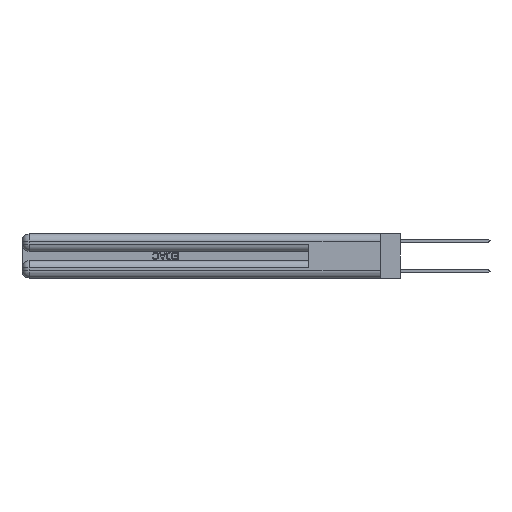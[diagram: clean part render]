
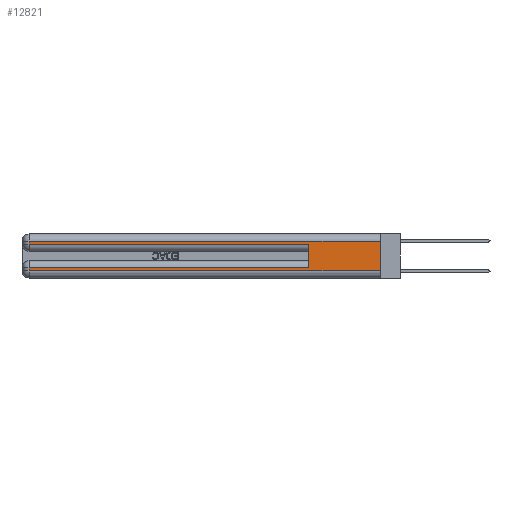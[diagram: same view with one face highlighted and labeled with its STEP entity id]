
A CAD part, left-side view. The second image highlights one B-rep face of the part: STEP entity #12821.
In plain terms, the highlighted planar face has unit normal (-1, 0, 0).
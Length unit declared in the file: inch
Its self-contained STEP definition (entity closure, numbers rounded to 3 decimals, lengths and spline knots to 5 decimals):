
#1538 = ORIENTED_EDGE ( 'NONE', *, *, #4470, .T. ) ;
#2518 = VERTEX_POINT ( 'NONE', #23135 ) ;
#2861 = VERTEX_POINT ( 'NONE', #29656 ) ;
#4069 = CARTESIAN_POINT ( 'NONE',  ( 0., 0., 0.06 ) ) ;
#4330 = DIRECTION ( 'NONE',  ( 0., -1., 0. ) ) ;
#4470 = EDGE_CURVE ( 'NONE', #31781, #13910, #30296, .T. ) ;
#4513 = CARTESIAN_POINT ( 'NONE',  ( 0., 0., 0.285 ) ) ;
#5048 = ORIENTED_EDGE ( 'NONE', *, *, #10285, .T. ) ;
#5128 = CARTESIAN_POINT ( 'NONE',  ( 0., 0., 0.06 ) ) ;
#5251 = ORIENTED_EDGE ( 'NONE', *, *, #26591, .F. ) ;
#5492 = DIRECTION ( 'NONE',  ( 0., 0., -1. ) ) ;
#5793 = ORIENTED_EDGE ( 'NONE', *, *, #26424, .T. ) ;
#5975 = FACE_OUTER_BOUND ( 'NONE', #10445, .T. ) ;
#6087 = LINE ( 'NONE', #33367, #21964 ) ;
#6448 = DIRECTION ( 'NONE',  ( 0., 1., 0. ) ) ;
#7720 = CARTESIAN_POINT ( 'NONE',  ( 0., 2.94, 0.31 ) ) ;
#8458 = PLANE ( 'NONE',  #12967 ) ;
#8974 = CARTESIAN_POINT ( 'NONE',  ( 0., 0.6, 0.285 ) ) ;
#8995 = EDGE_CURVE ( 'NONE', #2518, #31781, #30570, .T. ) ;
#9068 = EDGE_CURVE ( 'NONE', #13910, #26732, #9793, .T. ) ;
#9234 = CARTESIAN_POINT ( 'NONE',  ( 0., 0.6, 0.085 ) ) ;
#9793 = LINE ( 'NONE', #4513, #30836 ) ;
#10277 = EDGE_CURVE ( 'NONE', #2861, #21350, #22102, .T. ) ;
#10285 = EDGE_CURVE ( 'NONE', #30242, #2861, #6087, .T. ) ;
#10440 = DIRECTION ( 'NONE',  ( 0., 0., 1. ) ) ;
#10445 = EDGE_LOOP ( 'NONE', ( #5251, #25486, #1538, #22451, #24078, #5048, #30577, #5793 ) ) ;
#11769 = CARTESIAN_POINT ( 'NONE',  ( 0., 0., 0.37 ) ) ;
#12229 = CARTESIAN_POINT ( 'NONE',  ( 0., 2.94, 0.285 ) ) ;
#12821 = ADVANCED_FACE ( 'NONE', ( #5975 ), #8458, .F. ) ;
#12967 = AXIS2_PLACEMENT_3D ( 'NONE', #11769, #33254, #13726 ) ;
#13726 = DIRECTION ( 'NONE',  ( 0., 0., -1. ) ) ;
#13910 = VERTEX_POINT ( 'NONE', #12229 ) ;
#15384 = VECTOR ( 'NONE', #10440, 39.37008 ) ;
#15757 = EDGE_CURVE ( 'NONE', #30242, #26732, #32096, .T. ) ;
#16814 = DIRECTION ( 'NONE',  ( 0., 1., 0. ) ) ;
#17155 = DIRECTION ( 'NONE',  ( 0., 0., -1. ) ) ;
#17459 = VERTEX_POINT ( 'NONE', #5128 ) ;
#18529 = CARTESIAN_POINT ( 'NONE',  ( 0., 0.6, 0.145 ) ) ;
#20287 = VECTOR ( 'NONE', #23430, 39.37008 ) ;
#20439 = DIRECTION ( 'NONE',  ( 0., -1., 0. ) ) ;
#21315 = CARTESIAN_POINT ( 'NONE',  ( 0., 0., 0.37 ) ) ;
#21350 = VERTEX_POINT ( 'NONE', #24193 ) ;
#21964 = VECTOR ( 'NONE', #16814, 39.37008 ) ;
#22102 = LINE ( 'NONE', #30213, #33785 ) ;
#22451 = ORIENTED_EDGE ( 'NONE', *, *, #9068, .T. ) ;
#22723 = LINE ( 'NONE', #4069, #30981 ) ;
#22940 = VECTOR ( 'NONE', #6448, 39.37008 ) ;
#23135 = CARTESIAN_POINT ( 'NONE',  ( 0., 0., 0.31 ) ) ;
#23430 = DIRECTION ( 'NONE',  ( 0., 0., -1. ) ) ;
#23971 = LINE ( 'NONE', #21315, #20287 ) ;
#24078 = ORIENTED_EDGE ( 'NONE', *, *, #15757, .F. ) ;
#24193 = CARTESIAN_POINT ( 'NONE',  ( 0., 2.94, 0.06 ) ) ;
#25472 = CARTESIAN_POINT ( 'NONE',  ( 0., 0., 0.31 ) ) ;
#25486 = ORIENTED_EDGE ( 'NONE', *, *, #8995, .T. ) ;
#26424 = EDGE_CURVE ( 'NONE', #21350, #17459, #22723, .T. ) ;
#26591 = EDGE_CURVE ( 'NONE', #2518, #17459, #23971, .T. ) ;
#26732 = VERTEX_POINT ( 'NONE', #8974 ) ;
#29116 = VECTOR ( 'NONE', #5492, 39.37008 ) ;
#29622 = CARTESIAN_POINT ( 'NONE',  ( 0., 2.94, 0.37 ) ) ;
#29656 = CARTESIAN_POINT ( 'NONE',  ( 0., 2.94, 0.085 ) ) ;
#30213 = CARTESIAN_POINT ( 'NONE',  ( 0., 2.94, 0.37 ) ) ;
#30242 = VERTEX_POINT ( 'NONE', #9234 ) ;
#30296 = LINE ( 'NONE', #29622, #29116 ) ;
#30570 = LINE ( 'NONE', #25472, #22940 ) ;
#30577 = ORIENTED_EDGE ( 'NONE', *, *, #10277, .T. ) ;
#30836 = VECTOR ( 'NONE', #4330, 39.37008 ) ;
#30981 = VECTOR ( 'NONE', #20439, 39.37008 ) ;
#31781 = VERTEX_POINT ( 'NONE', #7720 ) ;
#32096 = LINE ( 'NONE', #18529, #15384 ) ;
#33254 = DIRECTION ( 'NONE',  ( 1., 0., 0. ) ) ;
#33367 = CARTESIAN_POINT ( 'NONE',  ( 0., 0., 0.085 ) ) ;
#33785 = VECTOR ( 'NONE', #17155, 39.37008 ) ;
